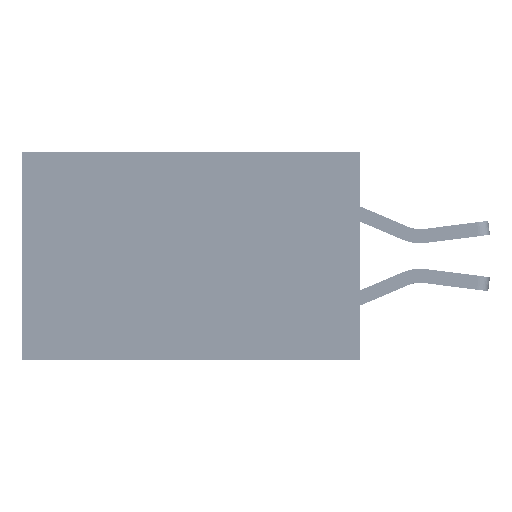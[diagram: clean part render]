
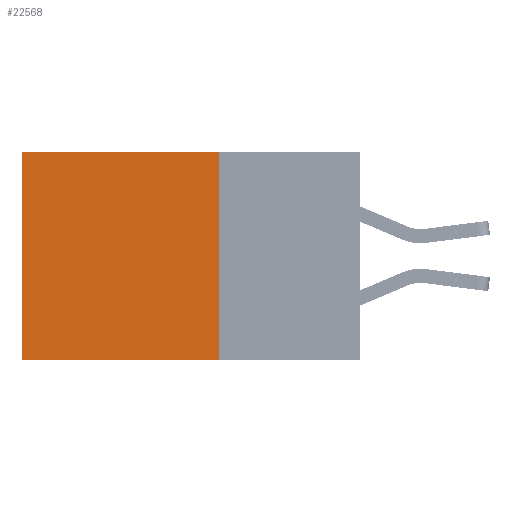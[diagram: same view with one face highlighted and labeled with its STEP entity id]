
A CAD part, left-side view. The second image highlights one B-rep face of the part: STEP entity #22568.
In plain terms, the highlighted planar face has unit normal (-1, 0, 0).
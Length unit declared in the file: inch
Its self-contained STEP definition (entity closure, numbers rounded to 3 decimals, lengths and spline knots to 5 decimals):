
#3805 = VERTEX_POINT ( 'NONE', #34763 ) ;
#3821 = ORIENTED_EDGE ( 'NONE', *, *, #36945, .T. ) ;
#5039 = VECTOR ( 'NONE', #13518, 39.37008 ) ;
#5087 = VERTEX_POINT ( 'NONE', #33112 ) ;
#5189 = DIRECTION ( 'NONE',  ( 1., 0., 0. ) ) ;
#5577 = VECTOR ( 'NONE', #30399, 39.37008 ) ;
#6982 = EDGE_CURVE ( 'NONE', #23295, #5087, #11292, .T. ) ;
#10325 = ORIENTED_EDGE ( 'NONE', *, *, #35548, .F. ) ;
#11292 = LINE ( 'NONE', #29232, #5039 ) ;
#11448 = CARTESIAN_POINT ( 'NONE',  ( 0.2875, 0.25, 0. ) ) ;
#13130 = DIRECTION ( 'NONE',  ( 0., 1., 0. ) ) ;
#13518 = DIRECTION ( 'NONE',  ( 0., 1., 0. ) ) ;
#14475 = FACE_OUTER_BOUND ( 'NONE', #39453, .T. ) ;
#17392 = VECTOR ( 'NONE', #13130, 39.37008 ) ;
#17601 = LINE ( 'NONE', #23971, #5577 ) ;
#18585 = VERTEX_POINT ( 'NONE', #29076 ) ;
#19662 = DIRECTION ( 'NONE',  ( 0., 0., -1. ) ) ;
#22141 = ORIENTED_EDGE ( 'NONE', *, *, #37714, .F. ) ;
#22309 = DIRECTION ( 'NONE',  ( 0., 0., -1. ) ) ;
#22568 = ADVANCED_FACE ( 'NONE', ( #14475 ), #24443, .F. ) ;
#22799 = VECTOR ( 'NONE', #22309, 39.37008 ) ;
#23295 = VERTEX_POINT ( 'NONE', #11448 ) ;
#23971 = CARTESIAN_POINT ( 'NONE',  ( 0.2875, 0.25, 0. ) ) ;
#24443 = PLANE ( 'NONE',  #33752 ) ;
#25831 = ORIENTED_EDGE ( 'NONE', *, *, #6982, .T. ) ;
#29076 = CARTESIAN_POINT ( 'NONE',  ( 0.2875, 0.25, -0.37 ) ) ;
#29232 = CARTESIAN_POINT ( 'NONE',  ( 0.2875, 0.25, 0. ) ) ;
#30399 = DIRECTION ( 'NONE',  ( 0., 0., -1. ) ) ;
#31532 = CARTESIAN_POINT ( 'NONE',  ( 0.2875, 0.25, -0.37 ) ) ;
#33112 = CARTESIAN_POINT ( 'NONE',  ( 0.2875, 0.6, 0. ) ) ;
#33510 = CARTESIAN_POINT ( 'NONE',  ( 0.2875, 0.25, 0. ) ) ;
#33752 = AXIS2_PLACEMENT_3D ( 'NONE', #33510, #5189, #19662 ) ;
#34763 = CARTESIAN_POINT ( 'NONE',  ( 0.2875, 0.6, -0.37 ) ) ;
#35548 = EDGE_CURVE ( 'NONE', #23295, #18585, #17601, .T. ) ;
#35605 = LINE ( 'NONE', #31532, #17392 ) ;
#36945 = EDGE_CURVE ( 'NONE', #5087, #3805, #37570, .T. ) ;
#37570 = LINE ( 'NONE', #37675, #22799 ) ;
#37675 = CARTESIAN_POINT ( 'NONE',  ( 0.2875, 0.6, 0. ) ) ;
#37714 = EDGE_CURVE ( 'NONE', #18585, #3805, #35605, .T. ) ;
#39453 = EDGE_LOOP ( 'NONE', ( #3821, #22141, #10325, #25831 ) ) ;
